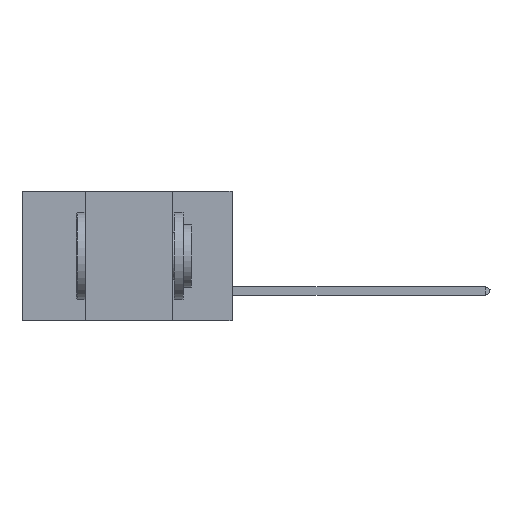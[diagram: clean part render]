
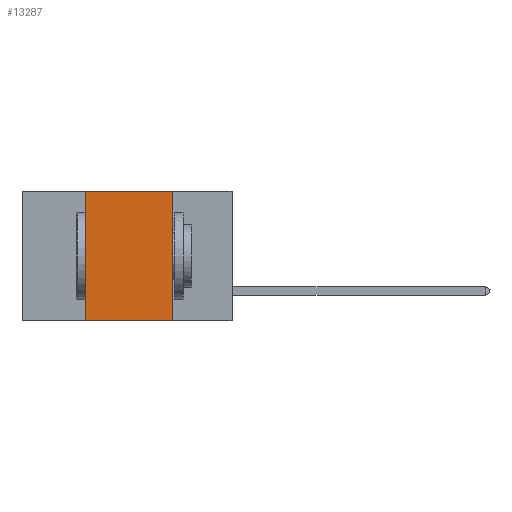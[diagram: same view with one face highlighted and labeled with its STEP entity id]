
A CAD part, left-side view. The second image highlights one B-rep face of the part: STEP entity #13287.
In plain terms, the highlighted planar face has unit normal (-1, 0, 0).
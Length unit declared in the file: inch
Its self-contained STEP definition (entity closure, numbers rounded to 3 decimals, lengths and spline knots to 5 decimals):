
#1438 = VERTEX_POINT ( 'NONE', #13910 ) ;
#1673 = DIRECTION ( 'NONE',  ( 0., 0., 1. ) ) ;
#1716 = VECTOR ( 'NONE', #25849, 39.37008 ) ;
#1858 = DIRECTION ( 'NONE',  ( 0., 0., -1. ) ) ;
#2066 = ORIENTED_EDGE ( 'NONE', *, *, #2162, .F. ) ;
#2162 = EDGE_CURVE ( 'NONE', #27928, #26998, #12783, .T. ) ;
#3555 = VERTEX_POINT ( 'NONE', #18375 ) ;
#4276 = VECTOR ( 'NONE', #20741, 39.37008 ) ;
#4773 = LINE ( 'NONE', #8952, #6478 ) ;
#6145 = PLANE ( 'NONE',  #25908 ) ;
#6478 = VECTOR ( 'NONE', #26584, 39.37008 ) ;
#8333 = CARTESIAN_POINT ( 'NONE',  ( 0., 0.17, 0. ) ) ;
#8336 = CARTESIAN_POINT ( 'NONE',  ( 0., 0.6, 0. ) ) ;
#8952 = CARTESIAN_POINT ( 'NONE',  ( 0., 0.6, -0.37 ) ) ;
#10441 = EDGE_CURVE ( 'NONE', #3555, #27928, #12131, .T. ) ;
#10879 = LINE ( 'NONE', #8333, #1716 ) ;
#11195 = ORIENTED_EDGE ( 'NONE', *, *, #17497, .T. ) ;
#12004 = CARTESIAN_POINT ( 'NONE',  ( 0., 0.17, 0. ) ) ;
#12131 = LINE ( 'NONE', #18742, #23681 ) ;
#12783 = LINE ( 'NONE', #20553, #4276 ) ;
#13287 = ADVANCED_FACE ( 'NONE', ( #24848 ), #6145, .F. ) ;
#13910 = CARTESIAN_POINT ( 'NONE',  ( 0., 0.17, -0.37 ) ) ;
#14962 = ORIENTED_EDGE ( 'NONE', *, *, #10441, .F. ) ;
#15443 = ORIENTED_EDGE ( 'NONE', *, *, #23480, .F. ) ;
#17497 = EDGE_CURVE ( 'NONE', #3555, #1438, #4773, .T. ) ;
#18375 = CARTESIAN_POINT ( 'NONE',  ( 0., 0.42, -0.37 ) ) ;
#18742 = CARTESIAN_POINT ( 'NONE',  ( 0., 0.42, 0. ) ) ;
#19251 = CARTESIAN_POINT ( 'NONE',  ( 0., 0.42, 0. ) ) ;
#20553 = CARTESIAN_POINT ( 'NONE',  ( 0., 0.6, 0. ) ) ;
#20741 = DIRECTION ( 'NONE',  ( 0., -1., 0. ) ) ;
#23480 = EDGE_CURVE ( 'NONE', #26998, #1438, #10879, .T. ) ;
#23681 = VECTOR ( 'NONE', #1673, 39.37008 ) ;
#24848 = FACE_OUTER_BOUND ( 'NONE', #25193, .T. ) ;
#25193 = EDGE_LOOP ( 'NONE', ( #15443, #2066, #14962, #11195 ) ) ;
#25671 = DIRECTION ( 'NONE',  ( 1., 0., 0. ) ) ;
#25849 = DIRECTION ( 'NONE',  ( 0., 0., -1. ) ) ;
#25908 = AXIS2_PLACEMENT_3D ( 'NONE', #8336, #25671, #1858 ) ;
#26584 = DIRECTION ( 'NONE',  ( 0., -1., 0. ) ) ;
#26998 = VERTEX_POINT ( 'NONE', #12004 ) ;
#27928 = VERTEX_POINT ( 'NONE', #19251 ) ;
